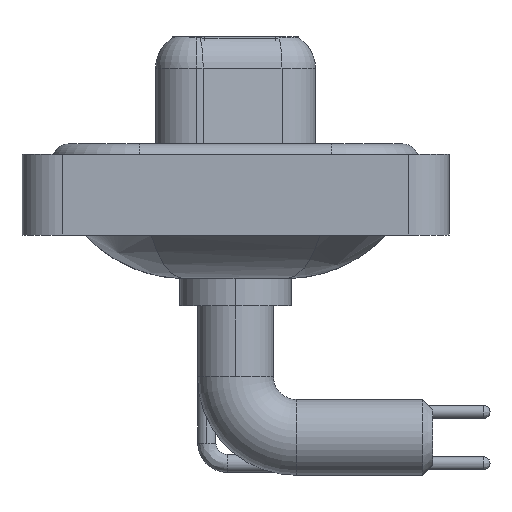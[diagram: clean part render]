
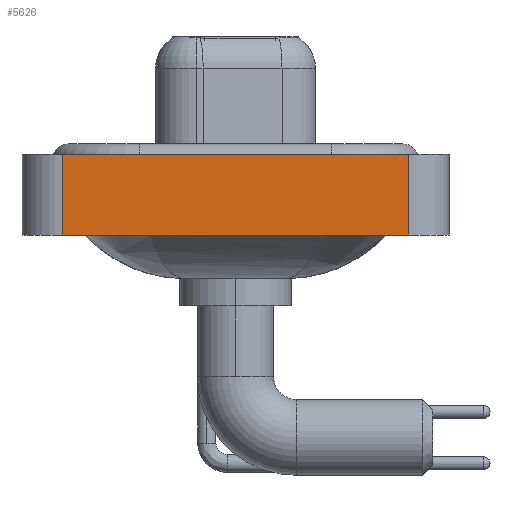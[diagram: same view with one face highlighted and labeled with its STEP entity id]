
A CAD part, left-side view. The second image highlights one B-rep face of the part: STEP entity #5626.
In plain terms, the highlighted planar face has unit normal (-1, 0, 0).
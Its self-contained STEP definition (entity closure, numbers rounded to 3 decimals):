
#93 = DIRECTION ( 'NONE',  ( 0., 0., 1. ) ) ;
#400 = LINE ( 'NONE', #1845, #9007 ) ;
#719 = VECTOR ( 'NONE', #14676, 1000. ) ;
#880 = VECTOR ( 'NONE', #15951, 1000. ) ;
#1845 = CARTESIAN_POINT ( 'NONE',  ( -7.3, -8.55, -3.6 ) ) ;
#2220 = CARTESIAN_POINT ( 'NONE',  ( -7.3, -8.55, -3.6 ) ) ;
#3661 = ORIENTED_EDGE ( 'NONE', *, *, #13413, .F. ) ;
#4625 = CARTESIAN_POINT ( 'NONE',  ( -7.3, 8.55, 0.4 ) ) ;
#5369 = VERTEX_POINT ( 'NONE', #18226 ) ;
#5626 = ADVANCED_FACE ( 'NONE', ( #10127 ), #11693, .T. ) ;
#6396 = CARTESIAN_POINT ( 'NONE',  ( -7.3, -8.55, 0.4 ) ) ;
#8455 = EDGE_LOOP ( 'NONE', ( #10119, #3661, #18329, #12742 ) ) ;
#9007 = VECTOR ( 'NONE', #93, 1000. ) ;
#9695 = LINE ( 'NONE', #15910, #719 ) ;
#10119 = ORIENTED_EDGE ( 'NONE', *, *, #16553, .T. ) ;
#10127 = FACE_OUTER_BOUND ( 'NONE', #8455, .T. ) ;
#11693 = PLANE ( 'NONE',  #11825 ) ;
#11825 = AXIS2_PLACEMENT_3D ( 'NONE', #16447, #16037, #17696 ) ;
#12077 = VERTEX_POINT ( 'NONE', #14557 ) ;
#12742 = ORIENTED_EDGE ( 'NONE', *, *, #19334, .T. ) ;
#13148 = VECTOR ( 'NONE', #17603, 1000. ) ;
#13413 = EDGE_CURVE ( 'NONE', #14742, #15228, #18858, .T. ) ;
#14557 = CARTESIAN_POINT ( 'NONE',  ( -7.3, 8.55, -3.6 ) ) ;
#14676 = DIRECTION ( 'NONE',  ( 0., 0., 1. ) ) ;
#14742 = VERTEX_POINT ( 'NONE', #4625 ) ;
#15228 = VERTEX_POINT ( 'NONE', #20462 ) ;
#15910 = CARTESIAN_POINT ( 'NONE',  ( -7.3, 8.55, -3.6 ) ) ;
#15951 = DIRECTION ( 'NONE',  ( 0., -1., 0. ) ) ;
#16037 = DIRECTION ( 'NONE',  ( -1., 0., 0. ) ) ;
#16447 = CARTESIAN_POINT ( 'NONE',  ( -7.3, -8.55, -3.6 ) ) ;
#16553 = EDGE_CURVE ( 'NONE', #5369, #15228, #400, .T. ) ;
#17603 = DIRECTION ( 'NONE',  ( 0., -1., 0. ) ) ;
#17696 = DIRECTION ( 'NONE',  ( 0., 0., 1. ) ) ;
#18226 = CARTESIAN_POINT ( 'NONE',  ( -7.3, -8.55, -3.6 ) ) ;
#18329 = ORIENTED_EDGE ( 'NONE', *, *, #18342, .F. ) ;
#18342 = EDGE_CURVE ( 'NONE', #12077, #14742, #9695, .T. ) ;
#18858 = LINE ( 'NONE', #6396, #880 ) ;
#19269 = LINE ( 'NONE', #2220, #13148 ) ;
#19334 = EDGE_CURVE ( 'NONE', #12077, #5369, #19269, .T. ) ;
#20462 = CARTESIAN_POINT ( 'NONE',  ( -7.3, -8.55, 0.4 ) ) ;
